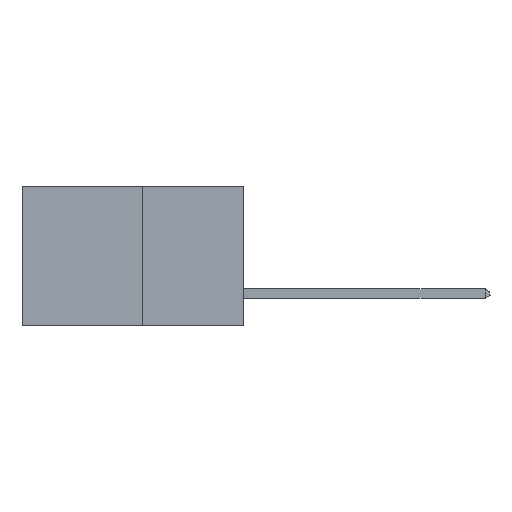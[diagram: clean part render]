
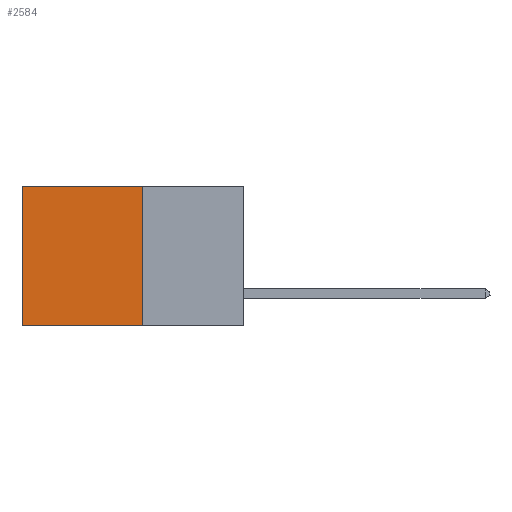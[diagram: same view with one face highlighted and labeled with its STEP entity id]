
A CAD part, left-side view. The second image highlights one B-rep face of the part: STEP entity #2584.
In plain terms, the highlighted planar face has unit normal (-1, 0, 0).
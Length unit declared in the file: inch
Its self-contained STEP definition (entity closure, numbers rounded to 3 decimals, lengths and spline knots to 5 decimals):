
#174 = EDGE_CURVE ( 'NONE', #3737, #5592, #5727, .T. ) ;
#260 = LINE ( 'NONE', #9440, #3011 ) ;
#514 = FACE_OUTER_BOUND ( 'NONE', #10821, .T. ) ;
#821 = DIRECTION ( 'NONE',  ( 0., 0., -1. ) ) ;
#2255 = VECTOR ( 'NONE', #3763, 39.37008 ) ;
#2532 = DIRECTION ( 'NONE',  ( 0., 1., 0. ) ) ;
#2584 = ADVANCED_FACE ( 'NONE', ( #514 ), #3393, .F. ) ;
#3011 = VECTOR ( 'NONE', #2532, 39.37008 ) ;
#3044 = DIRECTION ( 'NONE',  ( 0., 0., -1. ) ) ;
#3289 = CARTESIAN_POINT ( 'NONE',  ( 0.277, 0.59, 0. ) ) ;
#3393 = PLANE ( 'NONE',  #8167 ) ;
#3609 = ORIENTED_EDGE ( 'NONE', *, *, #10977, .F. ) ;
#3628 = VECTOR ( 'NONE', #821, 39.37008 ) ;
#3737 = VERTEX_POINT ( 'NONE', #3933 ) ;
#3763 = DIRECTION ( 'NONE',  ( 0., 0., -1. ) ) ;
#3805 = CARTESIAN_POINT ( 'NONE',  ( 0.277, 0.27, -0.37 ) ) ;
#3813 = VERTEX_POINT ( 'NONE', #5334 ) ;
#3933 = CARTESIAN_POINT ( 'NONE',  ( 0.277, 0.27, 0. ) ) ;
#4281 = CARTESIAN_POINT ( 'NONE',  ( 0.277, 0.27, -0.37 ) ) ;
#4805 = VECTOR ( 'NONE', #4810, 39.37008 ) ;
#4810 = DIRECTION ( 'NONE',  ( 0., 1., 0. ) ) ;
#5125 = LINE ( 'NONE', #3805, #4805 ) ;
#5334 = CARTESIAN_POINT ( 'NONE',  ( 0.277, 0.59, -0.37 ) ) ;
#5592 = VERTEX_POINT ( 'NONE', #11760 ) ;
#5727 = LINE ( 'NONE', #4281, #2255 ) ;
#6287 = LINE ( 'NONE', #7128, #3628 ) ;
#6944 = EDGE_CURVE ( 'NONE', #11407, #3813, #6287, .T. ) ;
#7040 = ORIENTED_EDGE ( 'NONE', *, *, #10883, .T. ) ;
#7128 = CARTESIAN_POINT ( 'NONE',  ( 0.277, 0.59, -0.37 ) ) ;
#7622 = ORIENTED_EDGE ( 'NONE', *, *, #174, .F. ) ;
#8167 = AXIS2_PLACEMENT_3D ( 'NONE', #9371, #12323, #3044 ) ;
#9371 = CARTESIAN_POINT ( 'NONE',  ( 0.277, 0.27, -0.37 ) ) ;
#9440 = CARTESIAN_POINT ( 'NONE',  ( 0.277, 0.27, 0. ) ) ;
#10821 = EDGE_LOOP ( 'NONE', ( #12169, #3609, #7622, #7040 ) ) ;
#10883 = EDGE_CURVE ( 'NONE', #3737, #11407, #260, .T. ) ;
#10977 = EDGE_CURVE ( 'NONE', #5592, #3813, #5125, .T. ) ;
#11407 = VERTEX_POINT ( 'NONE', #3289 ) ;
#11760 = CARTESIAN_POINT ( 'NONE',  ( 0.277, 0.27, -0.37 ) ) ;
#12169 = ORIENTED_EDGE ( 'NONE', *, *, #6944, .T. ) ;
#12323 = DIRECTION ( 'NONE',  ( 1., 0., 0. ) ) ;
